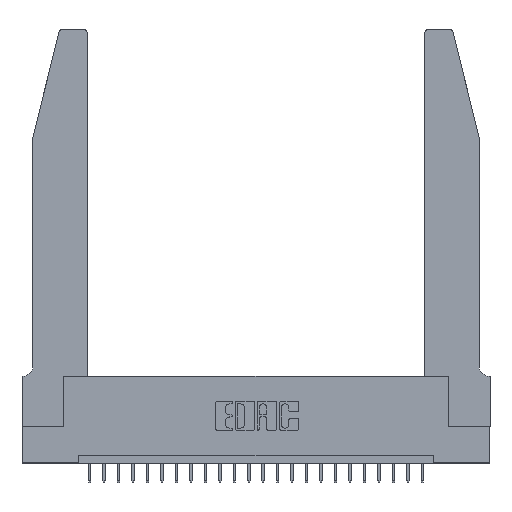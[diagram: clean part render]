
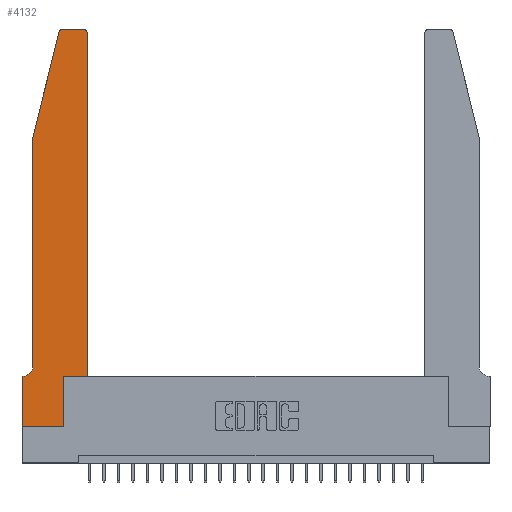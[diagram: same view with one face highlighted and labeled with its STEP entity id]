
A CAD part, top view. The second image highlights one B-rep face of the part: STEP entity #4132.
In plain terms, the highlighted planar face has unit normal (0, 0, 1).
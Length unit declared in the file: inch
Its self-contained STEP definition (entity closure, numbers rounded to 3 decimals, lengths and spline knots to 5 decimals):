
#246 = LINE ( 'NONE', #13608, #2258 ) ;
#323 = EDGE_CURVE ( 'NONE', #13439, #4878, #23170, .T. ) ;
#1029 = CARTESIAN_POINT ( 'NONE',  ( 0.0755, 2., 0.37 ) ) ;
#1120 = DIRECTION ( 'NONE',  ( 0., 0., -1. ) ) ;
#1666 = VERTEX_POINT ( 'NONE', #10084 ) ;
#1712 = VERTEX_POINT ( 'NONE', #5829 ) ;
#2011 = ORIENTED_EDGE ( 'NONE', *, *, #22709, .T. ) ;
#2131 = CIRCLE ( 'NONE', #12810, 0.03 ) ;
#2258 = VECTOR ( 'NONE', #4239, 39.37008 ) ;
#2291 = AXIS2_PLACEMENT_3D ( 'NONE', #14171, #17434, #23382 ) ;
#2410 = EDGE_CURVE ( 'NONE', #18013, #22495, #23789, .T. ) ;
#2433 = VERTEX_POINT ( 'NONE', #6511 ) ;
#2947 = LINE ( 'NONE', #1029, #16751 ) ;
#3204 = DIRECTION ( 'NONE',  ( 0., 1., 0. ) ) ;
#3541 = CARTESIAN_POINT ( 'NONE',  ( 0.4505, 0.35, 0.37 ) ) ;
#3693 = ORIENTED_EDGE ( 'NONE', *, *, #15083, .T. ) ;
#3956 = AXIS2_PLACEMENT_3D ( 'NONE', #20326, #1120, #14463 ) ;
#4132 = ADVANCED_FACE ( 'NONE', ( #5847 ), #6343, .T. ) ;
#4239 = DIRECTION ( 'NONE',  ( 1., 0., 0. ) ) ;
#4492 = EDGE_CURVE ( 'NONE', #10861, #13439, #20246, .T. ) ;
#4878 = VERTEX_POINT ( 'NONE', #18936 ) ;
#4915 = ORIENTED_EDGE ( 'NONE', *, *, #14457, .T. ) ;
#5110 = VERTEX_POINT ( 'NONE', #20991 ) ;
#5162 = DIRECTION ( 'NONE',  ( -0.239, -0.971, 0. ) ) ;
#5197 = DIRECTION ( 'NONE',  ( 0., -1., 0. ) ) ;
#5264 = ORIENTED_EDGE ( 'NONE', *, *, #15188, .T. ) ;
#5291 = CARTESIAN_POINT ( 'NONE',  ( 0.284, 2.72, 0.37 ) ) ;
#5635 = CIRCLE ( 'NONE', #21972, 0.03 ) ;
#5827 = DIRECTION ( 'NONE',  ( -1., 0., 0. ) ) ;
#5829 = CARTESIAN_POINT ( 'NONE',  ( 0.4205, 2.75, 0.37 ) ) ;
#5847 = FACE_OUTER_BOUND ( 'NONE', #22942, .T. ) ;
#5864 = ORIENTED_EDGE ( 'NONE', *, *, #6618, .T. ) ;
#6343 = PLANE ( 'NONE',  #2291 ) ;
#6465 = LINE ( 'NONE', #24535, #15145 ) ;
#6511 = CARTESIAN_POINT ( 'NONE',  ( 0.284, 2.75, 0.37 ) ) ;
#6618 = EDGE_CURVE ( 'NONE', #1666, #18013, #246, .T. ) ;
#7097 = LINE ( 'NONE', #14907, #10284 ) ;
#8469 = CARTESIAN_POINT ( 'NONE',  ( 0., 0., 0.37 ) ) ;
#8531 = VERTEX_POINT ( 'NONE', #9889 ) ;
#8703 = ORIENTED_EDGE ( 'NONE', *, *, #23702, .T. ) ;
#8885 = DIRECTION ( 'NONE',  ( 0., -1., 0. ) ) ;
#9008 = CARTESIAN_POINT ( 'NONE',  ( 0.2865, 0.35, 0.37 ) ) ;
#9743 = VECTOR ( 'NONE', #3204, 39.37008 ) ;
#9889 = CARTESIAN_POINT ( 'NONE',  ( 0., 0.35, 0.37 ) ) ;
#9922 = EDGE_CURVE ( 'NONE', #2433, #5110, #5635, .T. ) ;
#10084 = CARTESIAN_POINT ( 'NONE',  ( 0.2865, 0.35, 0.37 ) ) ;
#10284 = VECTOR ( 'NONE', #5197, 39.37008 ) ;
#10800 = DIRECTION ( 'NONE',  ( 0., 0., 1. ) ) ;
#10861 = VERTEX_POINT ( 'NONE', #12966 ) ;
#10968 = DIRECTION ( 'NONE',  ( -1., 0., 0. ) ) ;
#11941 = CARTESIAN_POINT ( 'NONE',  ( 0.4505, 2.72, 0.37 ) ) ;
#12049 = ORIENTED_EDGE ( 'NONE', *, *, #2410, .T. ) ;
#12810 = AXIS2_PLACEMENT_3D ( 'NONE', #20474, #10800, #18525 ) ;
#12966 = CARTESIAN_POINT ( 'NONE',  ( 0.0755, 2., 0.37 ) ) ;
#13126 = DIRECTION ( 'NONE',  ( 0., 0., 1. ) ) ;
#13163 = ORIENTED_EDGE ( 'NONE', *, *, #4492, .T. ) ;
#13439 = VERTEX_POINT ( 'NONE', #25145 ) ;
#13608 = CARTESIAN_POINT ( 'NONE',  ( 0.4505, 0.35, 0.37 ) ) ;
#13678 = EDGE_CURVE ( 'NONE', #5110, #10861, #2947, .T. ) ;
#13708 = CARTESIAN_POINT ( 'NONE',  ( 0.4505, 0.35, 0.37 ) ) ;
#14075 = DIRECTION ( 'NONE',  ( 0., 1., 0. ) ) ;
#14171 = CARTESIAN_POINT ( 'NONE',  ( 0., 0.35, 0.37 ) ) ;
#14294 = DIRECTION ( 'NONE',  ( 1., 0., 0. ) ) ;
#14457 = EDGE_CURVE ( 'NONE', #4878, #8531, #23081, .T. ) ;
#14463 = DIRECTION ( 'NONE',  ( -1., 0., 0. ) ) ;
#14491 = VECTOR ( 'NONE', #14075, 39.37008 ) ;
#14880 = CARTESIAN_POINT ( 'NONE',  ( 0.0755, 2., 0.37 ) ) ;
#14907 = CARTESIAN_POINT ( 'NONE',  ( 0., 0., 0.37 ) ) ;
#15083 = EDGE_CURVE ( 'NONE', #17352, #21525, #6465, .T. ) ;
#15145 = VECTOR ( 'NONE', #14294, 39.37008 ) ;
#15188 = EDGE_CURVE ( 'NONE', #8531, #17352, #7097, .T. ) ;
#15251 = DIRECTION ( 'NONE',  ( 1., 0., 0. ) ) ;
#15503 = VECTOR ( 'NONE', #10968, 39.37008 ) ;
#16250 = VECTOR ( 'NONE', #5827, 39.37008 ) ;
#16751 = VECTOR ( 'NONE', #5162, 39.37008 ) ;
#17260 = CARTESIAN_POINT ( 'NONE',  ( 0.0755, 0.35, 0.37 ) ) ;
#17346 = ORIENTED_EDGE ( 'NONE', *, *, #323, .T. ) ;
#17352 = VERTEX_POINT ( 'NONE', #8469 ) ;
#17434 = DIRECTION ( 'NONE',  ( 0., 0., 1. ) ) ;
#17637 = EDGE_CURVE ( 'NONE', #22495, #1712, #2131, .T. ) ;
#18013 = VERTEX_POINT ( 'NONE', #3541 ) ;
#18525 = DIRECTION ( 'NONE',  ( 1., 0., 0. ) ) ;
#18936 = CARTESIAN_POINT ( 'NONE',  ( 0.0055, 0.35, 0.37 ) ) ;
#19617 = CARTESIAN_POINT ( 'NONE',  ( 0.2605, 2.75, 0.37 ) ) ;
#20246 = LINE ( 'NONE', #14880, #22625 ) ;
#20326 = CARTESIAN_POINT ( 'NONE',  ( 0.0055, 0.42, 0.37 ) ) ;
#20474 = CARTESIAN_POINT ( 'NONE',  ( 0.4205, 2.72, 0.37 ) ) ;
#20991 = CARTESIAN_POINT ( 'NONE',  ( 0.25487, 2.72718, 0.37 ) ) ;
#21525 = VERTEX_POINT ( 'NONE', #24763 ) ;
#21691 = LINE ( 'NONE', #19617, #16250 ) ;
#21972 = AXIS2_PLACEMENT_3D ( 'NONE', #5291, #13126, #15251 ) ;
#22421 = LINE ( 'NONE', #9008, #9743 ) ;
#22441 = ORIENTED_EDGE ( 'NONE', *, *, #13678, .T. ) ;
#22495 = VERTEX_POINT ( 'NONE', #11941 ) ;
#22625 = VECTOR ( 'NONE', #8885, 39.37008 ) ;
#22709 = EDGE_CURVE ( 'NONE', #21525, #1666, #22421, .T. ) ;
#22942 = EDGE_LOOP ( 'NONE', ( #8703, #23159, #22441, #13163, #17346, #4915, #5264, #3693, #2011, #5864, #12049, #24317 ) ) ;
#23081 = LINE ( 'NONE', #17260, #15503 ) ;
#23159 = ORIENTED_EDGE ( 'NONE', *, *, #9922, .T. ) ;
#23170 = CIRCLE ( 'NONE', #3956, 0.07 ) ;
#23382 = DIRECTION ( 'NONE',  ( 1., 0., 0. ) ) ;
#23702 = EDGE_CURVE ( 'NONE', #1712, #2433, #21691, .T. ) ;
#23789 = LINE ( 'NONE', #13708, #14491 ) ;
#24317 = ORIENTED_EDGE ( 'NONE', *, *, #17637, .T. ) ;
#24535 = CARTESIAN_POINT ( 'NONE',  ( 0., 0., 0.37 ) ) ;
#24763 = CARTESIAN_POINT ( 'NONE',  ( 0.2865, 0., 0.37 ) ) ;
#25145 = CARTESIAN_POINT ( 'NONE',  ( 0.0755, 0.42, 0.37 ) ) ;
